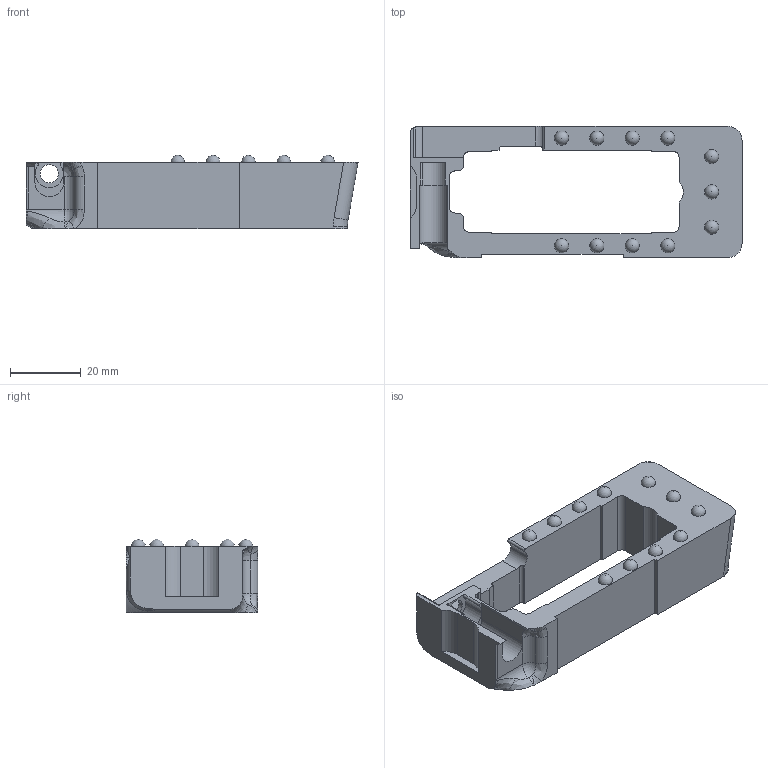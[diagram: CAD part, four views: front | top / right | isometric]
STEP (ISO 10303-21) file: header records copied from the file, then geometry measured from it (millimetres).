
FILE_DESCRIPTION (( 'STEP AP214' ), '1' );
FILE_NAME ('Magwell_2.STEP', '2013-09-01T16:47:06', ( 'Asher' ), ( '' ), 'SwSTEP 2.0', 'SolidWorks 2013', '' );
FILE_SCHEMA (( 'AUTOMOTIVE_DESIGN' ));
Length unit declared in the file: millimetre
Products named in the file (1): Magwell_2
Bounding box: 93.81 x 37.13 x 20.71 mm (x, y, z)
Volume: 30797.5 mm3; surface area: 11938.3 mm2
Topology: 1 solids, 1 shells, 120 faces, 349 edges, 230 vertices
Faces by surface type: cylinder 43, plane 42, bspline 16, sphere 13, torus 6
Entity records: 4851 total; most frequent: CARTESIAN_POINT 1467, ORIENTED_EDGE 652, DIRECTION 593, EDGE_CURVE 326, VERTEX_POINT 219, AXIS2_PLACEMENT_3D 217, VECTOR 159, LINE 159
